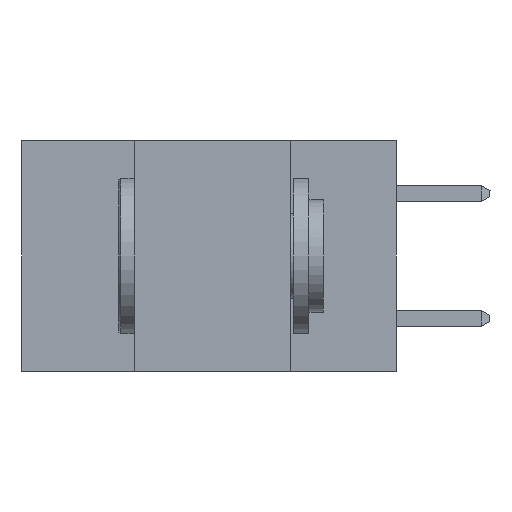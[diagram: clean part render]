
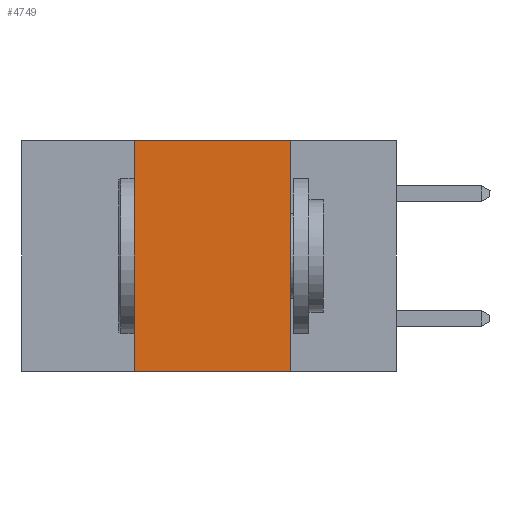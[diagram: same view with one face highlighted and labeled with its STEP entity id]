
A CAD part, left-side view. The second image highlights one B-rep face of the part: STEP entity #4749.
In plain terms, the highlighted planar face has unit normal (-1, 0, 0).
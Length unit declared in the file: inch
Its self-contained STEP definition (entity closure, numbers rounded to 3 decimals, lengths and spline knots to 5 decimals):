
#747 = DIRECTION ( 'NONE',  ( 0., 0., -1. ) ) ;
#1129 = DIRECTION ( 'NONE',  ( 1., 0., 0. ) ) ;
#1217 = ORIENTED_EDGE ( 'NONE', *, *, #5852, .F. ) ;
#1840 = LINE ( 'NONE', #5550, #11629 ) ;
#2247 = LINE ( 'NONE', #11747, #12033 ) ;
#3168 = EDGE_CURVE ( 'NONE', #11000, #4647, #8184, .T. ) ;
#3780 = CARTESIAN_POINT ( 'NONE',  ( 0., 0.17, 0. ) ) ;
#4268 = CARTESIAN_POINT ( 'NONE',  ( 0., 0.42, -0.37 ) ) ;
#4647 = VERTEX_POINT ( 'NONE', #7995 ) ;
#4749 = ADVANCED_FACE ( 'NONE', ( #11367 ), #6027, .F. ) ;
#4783 = ORIENTED_EDGE ( 'NONE', *, *, #3168, .F. ) ;
#5550 = CARTESIAN_POINT ( 'NONE',  ( 0., 0.6, 0. ) ) ;
#5713 = VECTOR ( 'NONE', #6640, 39.37008 ) ;
#5852 = EDGE_CURVE ( 'NONE', #12047, #8831, #2247, .T. ) ;
#5933 = CARTESIAN_POINT ( 'NONE',  ( 0., 0.6, -0.37 ) ) ;
#6027 = PLANE ( 'NONE',  #8787 ) ;
#6465 = DIRECTION ( 'NONE',  ( 0., -1., 0. ) ) ;
#6490 = CARTESIAN_POINT ( 'NONE',  ( 0., 0.17, 0. ) ) ;
#6640 = DIRECTION ( 'NONE',  ( 0., 0., -1. ) ) ;
#6813 = EDGE_LOOP ( 'NONE', ( #4783, #9670, #1217, #8708 ) ) ;
#6878 = DIRECTION ( 'NONE',  ( 0., -1., 0. ) ) ;
#7961 = EDGE_CURVE ( 'NONE', #8831, #11000, #1840, .T. ) ;
#7995 = CARTESIAN_POINT ( 'NONE',  ( 0., 0.17, -0.37 ) ) ;
#8148 = DIRECTION ( 'NONE',  ( 0., 0., 1. ) ) ;
#8184 = LINE ( 'NONE', #3780, #5713 ) ;
#8515 = CARTESIAN_POINT ( 'NONE',  ( 0., 0.6, 0. ) ) ;
#8708 = ORIENTED_EDGE ( 'NONE', *, *, #10564, .T. ) ;
#8787 = AXIS2_PLACEMENT_3D ( 'NONE', #8515, #1129, #747 ) ;
#8831 = VERTEX_POINT ( 'NONE', #10063 ) ;
#9670 = ORIENTED_EDGE ( 'NONE', *, *, #7961, .F. ) ;
#9747 = LINE ( 'NONE', #5933, #11847 ) ;
#10063 = CARTESIAN_POINT ( 'NONE',  ( 0., 0.42, 0. ) ) ;
#10564 = EDGE_CURVE ( 'NONE', #12047, #4647, #9747, .T. ) ;
#11000 = VERTEX_POINT ( 'NONE', #6490 ) ;
#11367 = FACE_OUTER_BOUND ( 'NONE', #6813, .T. ) ;
#11629 = VECTOR ( 'NONE', #6465, 39.37008 ) ;
#11747 = CARTESIAN_POINT ( 'NONE',  ( 0., 0.42, 0. ) ) ;
#11847 = VECTOR ( 'NONE', #6878, 39.37008 ) ;
#12033 = VECTOR ( 'NONE', #8148, 39.37008 ) ;
#12047 = VERTEX_POINT ( 'NONE', #4268 ) ;
